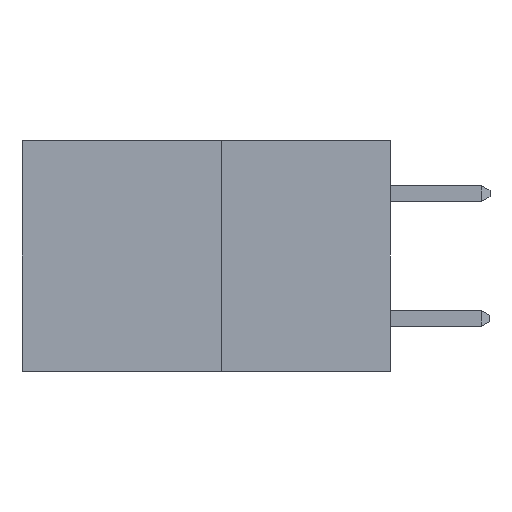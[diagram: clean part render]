
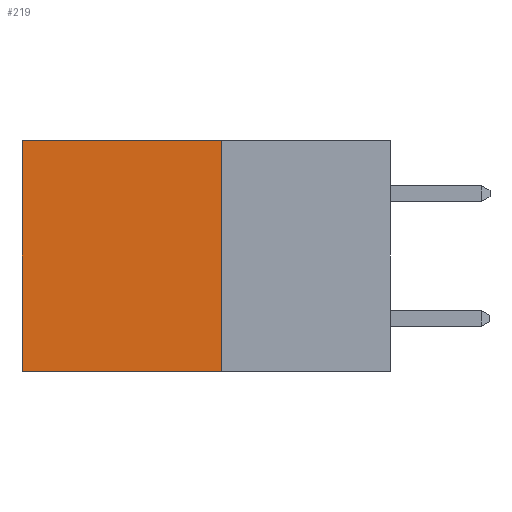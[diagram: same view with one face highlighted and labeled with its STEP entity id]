
A CAD part, left-side view. The second image highlights one B-rep face of the part: STEP entity #219.
In plain terms, the highlighted planar face has unit normal (-1, 0, 0).
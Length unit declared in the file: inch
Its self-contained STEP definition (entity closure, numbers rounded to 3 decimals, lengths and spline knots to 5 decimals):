
#219 = ADVANCED_FACE ( 'NONE', ( #2518 ), #3344, .F. ) ;
#564 = AXIS2_PLACEMENT_3D ( 'NONE', #7108, #3561, #3552 ) ;
#993 = ORIENTED_EDGE ( 'NONE', *, *, #2337, .T. ) ;
#1571 = CARTESIAN_POINT ( 'NONE',  ( 0.277, 0.27, -0.37 ) ) ;
#1606 = VECTOR ( 'NONE', #8437, 39.37008 ) ;
#1758 = LINE ( 'NONE', #4178, #5530 ) ;
#1856 = VERTEX_POINT ( 'NONE', #1571 ) ;
#2269 = CARTESIAN_POINT ( 'NONE',  ( 0.277, 0.27, -0.37 ) ) ;
#2294 = DIRECTION ( 'NONE',  ( 0., 0., -1. ) ) ;
#2337 = EDGE_CURVE ( 'NONE', #3660, #8093, #8808, .T. ) ;
#2389 = DIRECTION ( 'NONE',  ( 0., 1., 0. ) ) ;
#2395 = CARTESIAN_POINT ( 'NONE',  ( 0.277, 0.27, -0.37 ) ) ;
#2518 = FACE_OUTER_BOUND ( 'NONE', #7812, .T. ) ;
#2712 = CARTESIAN_POINT ( 'NONE',  ( 0.277, 0.59, 0. ) ) ;
#3002 = CARTESIAN_POINT ( 'NONE',  ( 0.277, 0.27, 0. ) ) ;
#3344 = PLANE ( 'NONE',  #564 ) ;
#3552 = DIRECTION ( 'NONE',  ( 0., 0., -1. ) ) ;
#3561 = DIRECTION ( 'NONE',  ( 1., 0., 0. ) ) ;
#3660 = VERTEX_POINT ( 'NONE', #8563 ) ;
#4178 = CARTESIAN_POINT ( 'NONE',  ( 0.277, 0.59, -0.37 ) ) ;
#4426 = CARTESIAN_POINT ( 'NONE',  ( 0.277, 0.59, -0.37 ) ) ;
#5130 = EDGE_CURVE ( 'NONE', #1856, #7148, #8239, .T. ) ;
#5199 = EDGE_CURVE ( 'NONE', #3660, #1856, #8763, .T. ) ;
#5530 = VECTOR ( 'NONE', #8289, 39.37008 ) ;
#5780 = VECTOR ( 'NONE', #2389, 39.37008 ) ;
#6938 = VECTOR ( 'NONE', #2294, 39.37008 ) ;
#6939 = EDGE_CURVE ( 'NONE', #8093, #7148, #1758, .T. ) ;
#7108 = CARTESIAN_POINT ( 'NONE',  ( 0.277, 0.27, -0.37 ) ) ;
#7148 = VERTEX_POINT ( 'NONE', #4426 ) ;
#7812 = EDGE_LOOP ( 'NONE', ( #8701, #7971, #8082, #993 ) ) ;
#7971 = ORIENTED_EDGE ( 'NONE', *, *, #5130, .F. ) ;
#8082 = ORIENTED_EDGE ( 'NONE', *, *, #5199, .F. ) ;
#8093 = VERTEX_POINT ( 'NONE', #2712 ) ;
#8239 = LINE ( 'NONE', #2395, #5780 ) ;
#8289 = DIRECTION ( 'NONE',  ( 0., 0., -1. ) ) ;
#8437 = DIRECTION ( 'NONE',  ( 0., 1., 0. ) ) ;
#8563 = CARTESIAN_POINT ( 'NONE',  ( 0.277, 0.27, 0. ) ) ;
#8701 = ORIENTED_EDGE ( 'NONE', *, *, #6939, .T. ) ;
#8763 = LINE ( 'NONE', #2269, #6938 ) ;
#8808 = LINE ( 'NONE', #3002, #1606 ) ;
